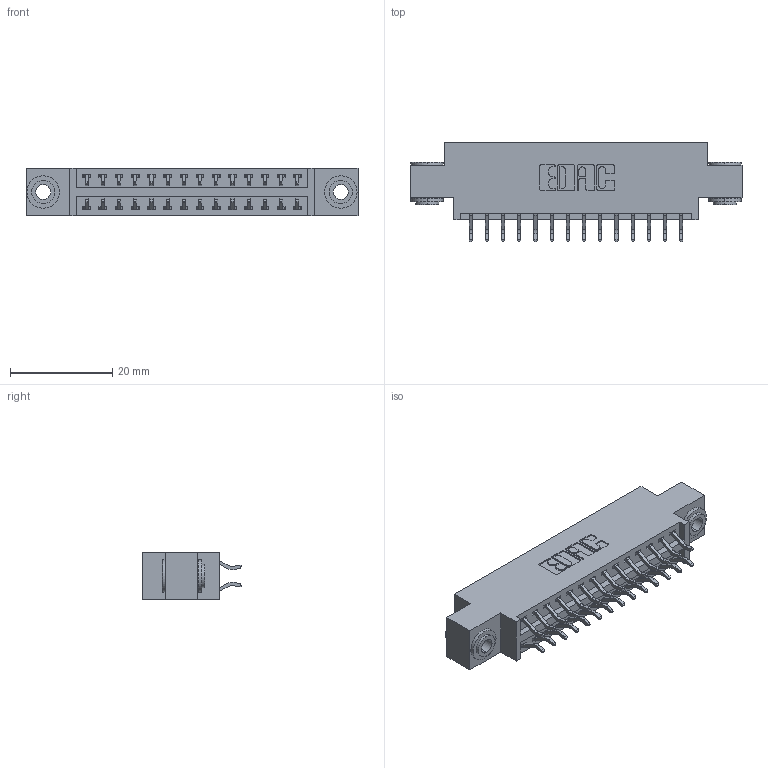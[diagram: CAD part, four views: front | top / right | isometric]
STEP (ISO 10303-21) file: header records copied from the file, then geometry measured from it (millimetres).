
FILE_DESCRIPTION (( 'STEP AP203' ), '1' );
FILE_NAME ('396-028-556-803.STEP', '2019-11-01T19:30:10', ( '' ), ( '' ), 'SwSTEP 2.0', 'SolidWorks 2016', '' );
FILE_SCHEMA (( 'CONFIG_CONTROL_DESIGN' ));
Length unit declared in the file: inch
Products named in the file (4): 346 Part_0.170 Offset - 0.156 Dia-TH; 345-292-001_556 Tail; 345-250-002_345-250-002-102; 396-028-556-803
Assembly tree (31 placements, depth 2):
  396-028-556-803
    346 Part_0.170 Offset - 0.156 Dia-TH
    345-292-001_556 Tail  x28
    345-250-002_345-250-002-102  x2
Bounding box: 65.02 x 19.57 x 9.4 mm (x, y, z)
Volume: 5986.9 mm3; surface area: 8157 mm2
Topology: 31 solids, 31 shells, 1788 faces, 5261 edges, 3466 vertices
Faces by surface type: plane 1182, cylinder 598, cone 8
Entity records: 13908 total; most frequent: CARTESIAN_POINT 2323, ORIENTED_EDGE 2238, DIRECTION 2117, EDGE_CURVE 1119, VECTOR 899, LINE 899, VERTEX_POINT 742, AXIS2_PLACEMENT_3D 609
